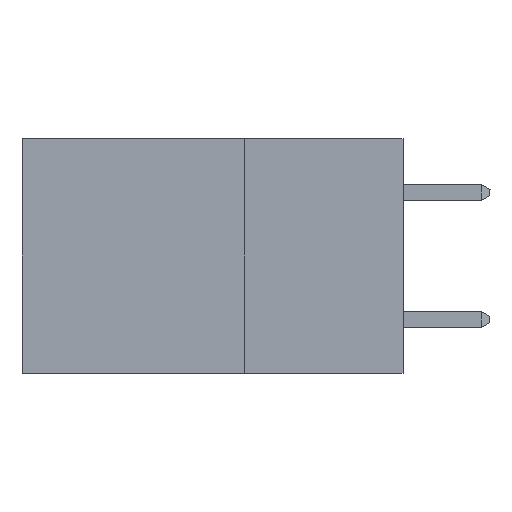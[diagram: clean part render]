
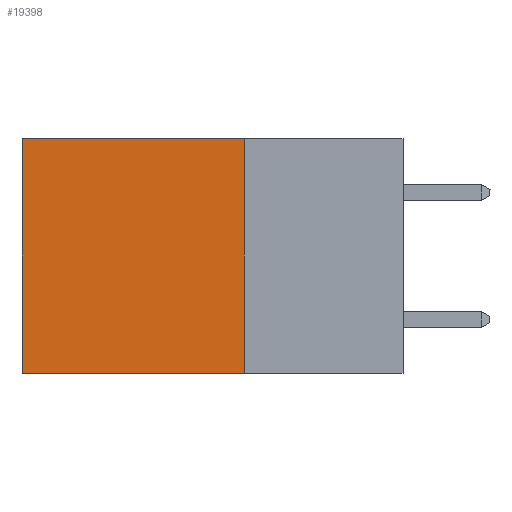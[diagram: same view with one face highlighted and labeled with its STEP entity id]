
A CAD part, left-side view. The second image highlights one B-rep face of the part: STEP entity #19398.
In plain terms, the highlighted planar face has unit normal (-1, 0, 0).
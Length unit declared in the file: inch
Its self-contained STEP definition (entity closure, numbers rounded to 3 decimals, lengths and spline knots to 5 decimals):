
#1644 = VECTOR ( 'NONE', #39111, 39.37008 ) ;
#1979 = EDGE_LOOP ( 'NONE', ( #6019, #11859, #27509, #22192 ) ) ;
#4396 = VERTEX_POINT ( 'NONE', #22142 ) ;
#4965 = CARTESIAN_POINT ( 'NONE',  ( 0.2875, 0.6, 0. ) ) ;
#6019 = ORIENTED_EDGE ( 'NONE', *, *, #20282, .T. ) ;
#6515 = CARTESIAN_POINT ( 'NONE',  ( 0.2875, 0.25, 0. ) ) ;
#7984 = VECTOR ( 'NONE', #14373, 39.37008 ) ;
#8059 = DIRECTION ( 'NONE',  ( 0., 0., -1. ) ) ;
#9500 = FACE_OUTER_BOUND ( 'NONE', #1979, .T. ) ;
#9602 = DIRECTION ( 'NONE',  ( 0., 0., -1. ) ) ;
#10140 = CARTESIAN_POINT ( 'NONE',  ( 0.2875, 0.25, 0. ) ) ;
#10434 = LINE ( 'NONE', #4965, #25651 ) ;
#11243 = LINE ( 'NONE', #22032, #35380 ) ;
#11859 = ORIENTED_EDGE ( 'NONE', *, *, #31464, .F. ) ;
#12570 = DIRECTION ( 'NONE',  ( 1., 0., 0. ) ) ;
#13976 = EDGE_CURVE ( 'NONE', #34414, #14730, #32216, .T. ) ;
#14373 = DIRECTION ( 'NONE',  ( 0., 0., -1. ) ) ;
#14730 = VERTEX_POINT ( 'NONE', #18435 ) ;
#15953 = DIRECTION ( 'NONE',  ( 0., 1., 0. ) ) ;
#16261 = VERTEX_POINT ( 'NONE', #17108 ) ;
#17108 = CARTESIAN_POINT ( 'NONE',  ( 0.2875, 0.6, -0.37 ) ) ;
#17447 = CARTESIAN_POINT ( 'NONE',  ( 0.2875, 0.25, 0. ) ) ;
#18435 = CARTESIAN_POINT ( 'NONE',  ( 0.2875, 0.25, -0.37 ) ) ;
#19398 = ADVANCED_FACE ( 'NONE', ( #9500 ), #24756, .F. ) ;
#20282 = EDGE_CURVE ( 'NONE', #4396, #16261, #10434, .T. ) ;
#22032 = CARTESIAN_POINT ( 'NONE',  ( 0.2875, 0.25, -0.37 ) ) ;
#22142 = CARTESIAN_POINT ( 'NONE',  ( 0.2875, 0.6, 0. ) ) ;
#22192 = ORIENTED_EDGE ( 'NONE', *, *, #34782, .T. ) ;
#24756 = PLANE ( 'NONE',  #31586 ) ;
#25651 = VECTOR ( 'NONE', #8059, 39.37008 ) ;
#27509 = ORIENTED_EDGE ( 'NONE', *, *, #13976, .F. ) ;
#31464 = EDGE_CURVE ( 'NONE', #14730, #16261, #11243, .T. ) ;
#31586 = AXIS2_PLACEMENT_3D ( 'NONE', #6515, #12570, #9602 ) ;
#32216 = LINE ( 'NONE', #17447, #7984 ) ;
#33682 = CARTESIAN_POINT ( 'NONE',  ( 0.2875, 0.25, 0. ) ) ;
#33998 = LINE ( 'NONE', #33682, #1644 ) ;
#34414 = VERTEX_POINT ( 'NONE', #10140 ) ;
#34782 = EDGE_CURVE ( 'NONE', #34414, #4396, #33998, .T. ) ;
#35380 = VECTOR ( 'NONE', #15953, 39.37008 ) ;
#39111 = DIRECTION ( 'NONE',  ( 0., 1., 0. ) ) ;
